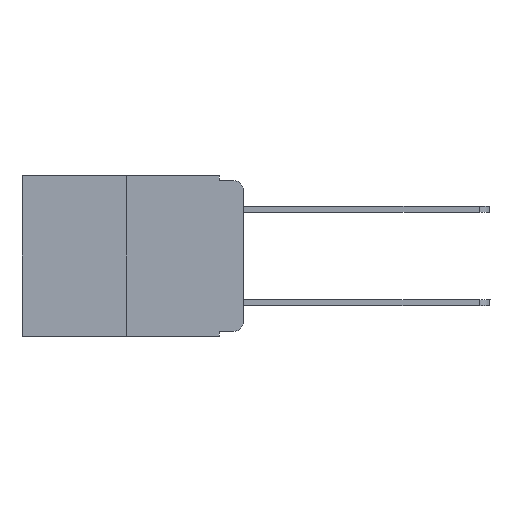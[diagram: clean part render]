
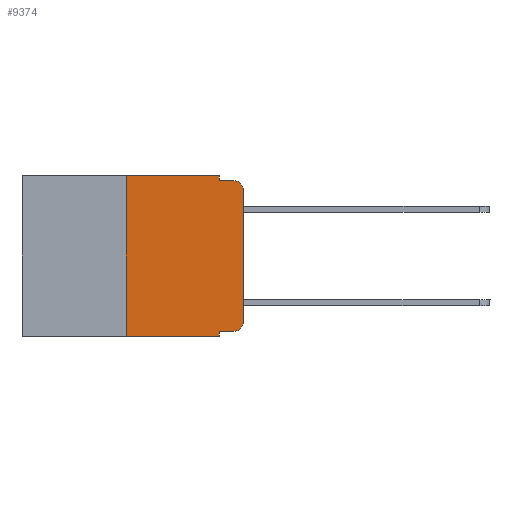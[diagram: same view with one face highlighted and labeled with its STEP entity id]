
A CAD part, left-side view. The second image highlights one B-rep face of the part: STEP entity #9374.
In plain terms, the highlighted planar face has unit normal (-1, 0, 0).
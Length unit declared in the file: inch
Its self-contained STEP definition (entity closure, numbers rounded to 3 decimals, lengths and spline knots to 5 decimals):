
#15 = ORIENTED_EDGE ( 'NONE', *, *, #10645, .F. ) ;
#176 = LINE ( 'NONE', #6034, #2915 ) ;
#276 = CARTESIAN_POINT ( 'NONE',  ( 0., 0.051, -0.01 ) ) ;
#701 = CARTESIAN_POINT ( 'NONE',  ( 0., 0.02, -0.333 ) ) ;
#709 = AXIS2_PLACEMENT_3D ( 'NONE', #4159, #8433, #10082 ) ;
#819 = CARTESIAN_POINT ( 'NONE',  ( 0., 0.051, -0.01 ) ) ;
#970 = EDGE_CURVE ( 'NONE', #6392, #5703, #176, .T. ) ;
#1020 = VERTEX_POINT ( 'NONE', #1922 ) ;
#1030 = VECTOR ( 'NONE', #2925, 39.37008 ) ;
#1110 = ORIENTED_EDGE ( 'NONE', *, *, #3253, .F. ) ;
#1530 = ORIENTED_EDGE ( 'NONE', *, *, #6880, .F. ) ;
#1799 = AXIS2_PLACEMENT_3D ( 'NONE', #8926, #8817, #7205 ) ;
#1922 = CARTESIAN_POINT ( 'NONE',  ( 0., 0.051, -0.343 ) ) ;
#2049 = CARTESIAN_POINT ( 'NONE',  ( 0., 0.02, -0.313 ) ) ;
#2255 = VECTOR ( 'NONE', #6344, 39.37008 ) ;
#2379 = DIRECTION ( 'NONE',  ( 0., -1., 0. ) ) ;
#2407 = LINE ( 'NONE', #5896, #8322 ) ;
#2429 = VERTEX_POINT ( 'NONE', #4765 ) ;
#2717 = LINE ( 'NONE', #6065, #7457 ) ;
#2915 = VECTOR ( 'NONE', #6860, 39.37008 ) ;
#2925 = DIRECTION ( 'NONE',  ( 0., -1., 0. ) ) ;
#2930 = VERTEX_POINT ( 'NONE', #3012 ) ;
#3012 = CARTESIAN_POINT ( 'NONE',  ( 0., 0., -0.313 ) ) ;
#3179 = CARTESIAN_POINT ( 'NONE',  ( 0., 0.051, -0.333 ) ) ;
#3253 = EDGE_CURVE ( 'NONE', #7999, #1020, #8077, .T. ) ;
#3361 = DIRECTION ( 'NONE',  ( 0., -1., 0. ) ) ;
#3443 = PLANE ( 'NONE',  #709 ) ;
#3546 = CARTESIAN_POINT ( 'NONE',  ( 0., 0.25, 0. ) ) ;
#3561 = VECTOR ( 'NONE', #2379, 39.37008 ) ;
#3572 = EDGE_CURVE ( 'NONE', #7999, #4420, #3800, .T. ) ;
#3800 = LINE ( 'NONE', #8105, #1030 ) ;
#4159 = CARTESIAN_POINT ( 'NONE',  ( 0., 0.473, 0. ) ) ;
#4194 = DIRECTION ( 'NONE',  ( 0., 0., 1. ) ) ;
#4205 = CARTESIAN_POINT ( 'NONE',  ( 0., 0.051, 0. ) ) ;
#4248 = ORIENTED_EDGE ( 'NONE', *, *, #3572, .T. ) ;
#4254 = LINE ( 'NONE', #3546, #9908 ) ;
#4420 = VERTEX_POINT ( 'NONE', #701 ) ;
#4434 = VERTEX_POINT ( 'NONE', #9075 ) ;
#4501 = EDGE_LOOP ( 'NONE', ( #6760, #8947, #15, #1530, #10227, #5564, #5287, #1110, #4248, #6992 ) ) ;
#4765 = CARTESIAN_POINT ( 'NONE',  ( 0., 0., -0.03 ) ) ;
#5046 = FACE_OUTER_BOUND ( 'NONE', #4501, .T. ) ;
#5058 = EDGE_CURVE ( 'NONE', #9125, #6392, #4254, .T. ) ;
#5101 = CARTESIAN_POINT ( 'NONE',  ( 0., 0.25, 0. ) ) ;
#5150 = DIRECTION ( 'NONE',  ( 0., 0., -1. ) ) ;
#5287 = ORIENTED_EDGE ( 'NONE', *, *, #5557, .T. ) ;
#5524 = CARTESIAN_POINT ( 'NONE',  ( 0., 0.051, 0. ) ) ;
#5557 = EDGE_CURVE ( 'NONE', #9125, #1020, #2717, .T. ) ;
#5564 = ORIENTED_EDGE ( 'NONE', *, *, #5058, .F. ) ;
#5703 = VERTEX_POINT ( 'NONE', #7462 ) ;
#5856 = LINE ( 'NONE', #4205, #6468 ) ;
#5896 = CARTESIAN_POINT ( 'NONE',  ( 0., 0., 0. ) ) ;
#6034 = CARTESIAN_POINT ( 'NONE',  ( 0., 0.473, 0. ) ) ;
#6065 = CARTESIAN_POINT ( 'NONE',  ( 0., 0.473, -0.343 ) ) ;
#6083 = EDGE_CURVE ( 'NONE', #4420, #2930, #7494, .T. ) ;
#6266 = CARTESIAN_POINT ( 'NONE',  ( 0., 0.25, -0.343 ) ) ;
#6344 = DIRECTION ( 'NONE',  ( 0., 0., -1. ) ) ;
#6392 = VERTEX_POINT ( 'NONE', #5101 ) ;
#6468 = VECTOR ( 'NONE', #5150, 39.37008 ) ;
#6760 = ORIENTED_EDGE ( 'NONE', *, *, #9780, .T. ) ;
#6860 = DIRECTION ( 'NONE',  ( 0., -1., 0. ) ) ;
#6876 = VERTEX_POINT ( 'NONE', #276 ) ;
#6880 = EDGE_CURVE ( 'NONE', #5703, #6876, #5856, .T. ) ;
#6992 = ORIENTED_EDGE ( 'NONE', *, *, #6083, .T. ) ;
#7205 = DIRECTION ( 'NONE',  ( 0., 0., -1. ) ) ;
#7457 = VECTOR ( 'NONE', #3361, 39.37008 ) ;
#7462 = CARTESIAN_POINT ( 'NONE',  ( 0., 0.051, 0. ) ) ;
#7494 = CIRCLE ( 'NONE', #9960, 0.02 ) ;
#7646 = DIRECTION ( 'NONE',  ( 0., 0., 1. ) ) ;
#7999 = VERTEX_POINT ( 'NONE', #3179 ) ;
#8077 = LINE ( 'NONE', #5524, #2255 ) ;
#8105 = CARTESIAN_POINT ( 'NONE',  ( 0., 0.051, -0.333 ) ) ;
#8322 = VECTOR ( 'NONE', #4194, 39.37008 ) ;
#8433 = DIRECTION ( 'NONE',  ( 1., 0., 0. ) ) ;
#8678 = DIRECTION ( 'NONE',  ( -1., 0., 0. ) ) ;
#8735 = EDGE_CURVE ( 'NONE', #2429, #4434, #10460, .T. ) ;
#8817 = DIRECTION ( 'NONE',  ( -1., 0., 0. ) ) ;
#8910 = DIRECTION ( 'NONE',  ( 0., 0., -1. ) ) ;
#8926 = CARTESIAN_POINT ( 'NONE',  ( 0., 0.02, -0.03 ) ) ;
#8947 = ORIENTED_EDGE ( 'NONE', *, *, #8735, .T. ) ;
#9075 = CARTESIAN_POINT ( 'NONE',  ( 0., 0.02, -0.01 ) ) ;
#9125 = VERTEX_POINT ( 'NONE', #6266 ) ;
#9374 = ADVANCED_FACE ( 'NONE', ( #5046 ), #3443, .F. ) ;
#9780 = EDGE_CURVE ( 'NONE', #2930, #2429, #2407, .T. ) ;
#9908 = VECTOR ( 'NONE', #7646, 39.37008 ) ;
#9960 = AXIS2_PLACEMENT_3D ( 'NONE', #2049, #8678, #8910 ) ;
#10042 = LINE ( 'NONE', #819, #3561 ) ;
#10082 = DIRECTION ( 'NONE',  ( 0., 0., -1. ) ) ;
#10227 = ORIENTED_EDGE ( 'NONE', *, *, #970, .F. ) ;
#10460 = CIRCLE ( 'NONE', #1799, 0.02 ) ;
#10645 = EDGE_CURVE ( 'NONE', #6876, #4434, #10042, .T. ) ;
